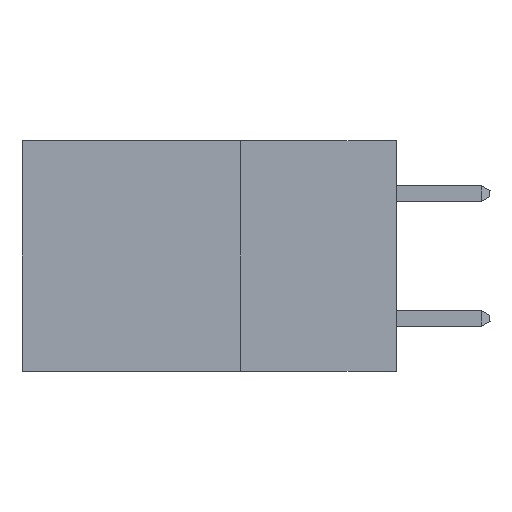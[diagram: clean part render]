
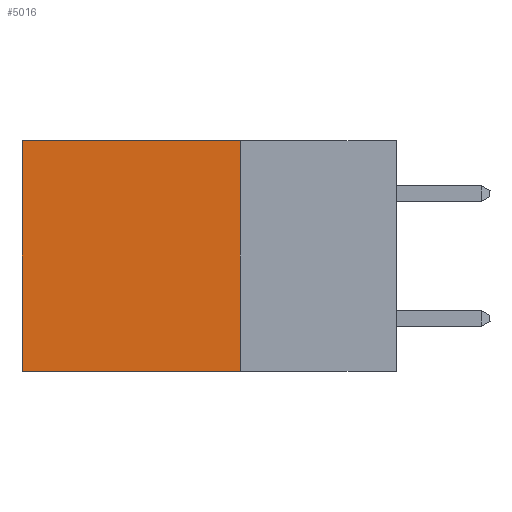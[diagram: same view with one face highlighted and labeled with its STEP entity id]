
A CAD part, left-side view. The second image highlights one B-rep face of the part: STEP entity #5016.
In plain terms, the highlighted planar face has unit normal (-1, 0, 0).
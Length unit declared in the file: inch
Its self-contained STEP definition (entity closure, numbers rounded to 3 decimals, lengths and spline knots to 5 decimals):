
#634 = CARTESIAN_POINT ( 'NONE',  ( 0.298, 0.25, 0. ) ) ;
#2572 = VERTEX_POINT ( 'NONE', #10702 ) ;
#3058 = LINE ( 'NONE', #12034, #20900 ) ;
#5016 = ADVANCED_FACE ( 'NONE', ( #25837 ), #21693, .F. ) ;
#5440 = VECTOR ( 'NONE', #13501, 39.37008 ) ;
#5784 = EDGE_CURVE ( 'NONE', #15065, #21130, #24155, .T. ) ;
#6180 = EDGE_LOOP ( 'NONE', ( #13063, #7039, #7360, #15910 ) ) ;
#7039 = ORIENTED_EDGE ( 'NONE', *, *, #5784, .F. ) ;
#7360 = ORIENTED_EDGE ( 'NONE', *, *, #25848, .F. ) ;
#9635 = EDGE_CURVE ( 'NONE', #2572, #14914, #21329, .T. ) ;
#10702 = CARTESIAN_POINT ( 'NONE',  ( 0.298, 0.25, 0. ) ) ;
#12034 = CARTESIAN_POINT ( 'NONE',  ( 0.298, 0.6, 0. ) ) ;
#12079 = CARTESIAN_POINT ( 'NONE',  ( 0.298, 0.25, 0. ) ) ;
#12198 = DIRECTION ( 'NONE',  ( 0., 1., 0. ) ) ;
#13063 = ORIENTED_EDGE ( 'NONE', *, *, #13699, .T. ) ;
#13501 = DIRECTION ( 'NONE',  ( 0., 1., 0. ) ) ;
#13699 = EDGE_CURVE ( 'NONE', #14914, #21130, #3058, .T. ) ;
#14232 = DIRECTION ( 'NONE',  ( 0., 0., -1. ) ) ;
#14914 = VERTEX_POINT ( 'NONE', #24468 ) ;
#15065 = VERTEX_POINT ( 'NONE', #19017 ) ;
#15712 = DIRECTION ( 'NONE',  ( 0., 0., -1. ) ) ;
#15910 = ORIENTED_EDGE ( 'NONE', *, *, #9635, .T. ) ;
#16439 = VECTOR ( 'NONE', #14232, 39.37008 ) ;
#17505 = CARTESIAN_POINT ( 'NONE',  ( 0.298, 0.25, 0. ) ) ;
#17567 = DIRECTION ( 'NONE',  ( 1., 0., 0. ) ) ;
#18350 = CARTESIAN_POINT ( 'NONE',  ( 0.298, 0.6, -0.37 ) ) ;
#19017 = CARTESIAN_POINT ( 'NONE',  ( 0.298, 0.25, -0.37 ) ) ;
#20900 = VECTOR ( 'NONE', #24978, 39.37008 ) ;
#21130 = VERTEX_POINT ( 'NONE', #18350 ) ;
#21329 = LINE ( 'NONE', #17505, #5440 ) ;
#21693 = PLANE ( 'NONE',  #23860 ) ;
#22923 = CARTESIAN_POINT ( 'NONE',  ( 0.298, 0.25, -0.37 ) ) ;
#23860 = AXIS2_PLACEMENT_3D ( 'NONE', #634, #17567, #15712 ) ;
#24155 = LINE ( 'NONE', #22923, #26819 ) ;
#24468 = CARTESIAN_POINT ( 'NONE',  ( 0.298, 0.6, 0. ) ) ;
#24978 = DIRECTION ( 'NONE',  ( 0., 0., -1. ) ) ;
#24991 = LINE ( 'NONE', #12079, #16439 ) ;
#25837 = FACE_OUTER_BOUND ( 'NONE', #6180, .T. ) ;
#25848 = EDGE_CURVE ( 'NONE', #2572, #15065, #24991, .T. ) ;
#26819 = VECTOR ( 'NONE', #12198, 39.37008 ) ;
